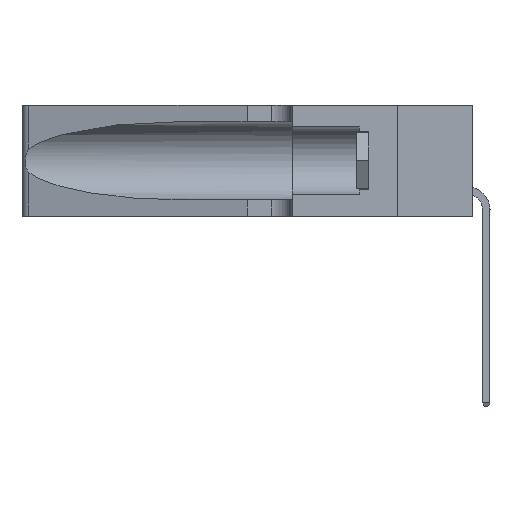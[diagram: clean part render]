
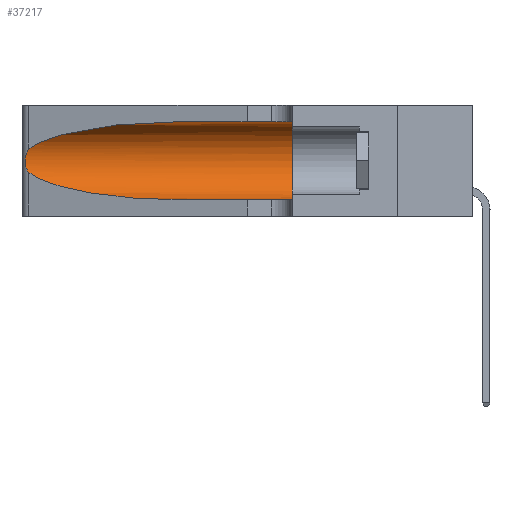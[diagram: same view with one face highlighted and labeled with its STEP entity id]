
A CAD part, left-side view. The second image highlights one B-rep face of the part: STEP entity #37217.
In plain terms, the highlighted cylindrical face has radius 3.308 mm (diameter 6.617 mm), a partial arc.
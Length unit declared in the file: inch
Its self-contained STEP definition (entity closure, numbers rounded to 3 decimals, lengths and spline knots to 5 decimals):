
#24 = CARTESIAN_POINT ( 'NONE',  ( 0.26075, 1.23896, 0.178 ) ) ;
#70 = CIRCLE ( 'NONE', #18635, 0.13025 ) ;
#520 = CARTESIAN_POINT ( 'NONE',  ( 0.1305, 1.61858, 0.31525 ) ) ;
#1106 = EDGE_CURVE ( 'NONE', #28408, #10484, #18541, .T. ) ;
#4346 = CARTESIAN_POINT ( 'NONE',  ( 0.18966, 0.96281, 0.31525 ) ) ;
#6622 = CARTESIAN_POINT ( 'NONE',  ( 0.1305, 0.35, 0.185 ) ) ;
#6805 = CARTESIAN_POINT ( 'NONE',  ( 0.25856, 1.23593, 0.16098 ) ) ;
#6912 = VERTEX_POINT ( 'NONE', #30365 ) ;
#6955 = CARTESIAN_POINT ( 'NONE',  ( 0.25487, 1.22718, 0.22369 ) ) ;
#7451 =( BOUNDED_CURVE ( )  B_SPLINE_CURVE ( 3, ( #17604, #4346, #10817, #21146 ),
 .UNSPECIFIED., .F., .F. ) 
 B_SPLINE_CURVE_WITH_KNOTS ( ( 4, 4 ),
 ( 1.5708, 2.84003 ),
 .UNSPECIFIED. ) 
 CURVE ( )  GEOMETRIC_REPRESENTATION_ITEM ( )  RATIONAL_B_SPLINE_CURVE ( ( 1., 0.87, 0.87, 1. ) ) 
 REPRESENTATION_ITEM ( '' )  );
#8233 = EDGE_CURVE ( 'NONE', #16642, #6912, #14654, .T. ) ;
#8557 =( BOUNDED_CURVE ( )  B_SPLINE_CURVE ( 3, ( #23113, #22842, #19428, #39682 ),
 .UNSPECIFIED., .F., .F. ) 
 B_SPLINE_CURVE_WITH_KNOTS ( ( 4, 4 ),
 ( 3.44316, 4.71239 ),
 .UNSPECIFIED. ) 
 CURVE ( )  GEOMETRIC_REPRESENTATION_ITEM ( )  RATIONAL_B_SPLINE_CURVE ( ( 1., 0.87, 0.87, 1. ) ) 
 REPRESENTATION_ITEM ( '' )  );
#9288 = CARTESIAN_POINT ( 'NONE',  ( 0.1305, 0.72297, 0.05475 ) ) ;
#10182 = CARTESIAN_POINT ( 'NONE',  ( 0.25555, 1.22993, 0.14849 ) ) ;
#10318 = CARTESIAN_POINT ( 'NONE',  ( 0.26018, 1.23835, 0.19895 ) ) ;
#10484 = VERTEX_POINT ( 'NONE', #36836 ) ;
#10817 = CARTESIAN_POINT ( 'NONE',  ( 0.2373, 1.15595, 0.28018 ) ) ;
#13384 = DIRECTION ( 'NONE',  ( 0., 0., 1. ) ) ;
#13590 = CARTESIAN_POINT ( 'NONE',  ( 0.25487, 1.22718, 0.14631 ) ) ;
#14347 = EDGE_CURVE ( 'NONE', #10484, #32507, #8557, .T. ) ;
#14654 = LINE ( 'NONE', #520, #37379 ) ;
#14724 = LINE ( 'NONE', #24856, #25330 ) ;
#16642 = VERTEX_POINT ( 'NONE', #31233 ) ;
#16738 = EDGE_CURVE ( 'NONE', #32507, #36580, #14724, .T. ) ;
#17604 = CARTESIAN_POINT ( 'NONE',  ( 0.1305, 0.72297, 0.31525 ) ) ;
#18541 = B_SPLINE_CURVE_WITH_KNOTS ( 'NONE', 3,
 ( #6955, #26858, #20503, #30702, #33678, #10318, #37094, #24, #23620, #6805, #43572, #30428, #10182, #13590 ),
 .UNSPECIFIED., .F., .F.,
 ( 4, 2, 2, 2, 2, 2, 4 ),
 ( 0., 0.00027, 0.00053, 0.00107, 0.0016, 0.00187, 0.00214 ),
 .UNSPECIFIED. ) ;
#18635 = AXIS2_PLACEMENT_3D ( 'NONE', #6622, #30216, #13384 ) ;
#19428 = CARTESIAN_POINT ( 'NONE',  ( 0.18966, 0.96281, 0.05475 ) ) ;
#19536 = CARTESIAN_POINT ( 'NONE',  ( 0.25487, 1.22718, 0.22369 ) ) ;
#20503 = CARTESIAN_POINT ( 'NONE',  ( 0.25639, 1.23184, 0.21858 ) ) ;
#20511 = ORIENTED_EDGE ( 'NONE', *, *, #8233, .F. ) ;
#21146 = CARTESIAN_POINT ( 'NONE',  ( 0.25487, 1.22718, 0.22369 ) ) ;
#21845 = EDGE_CURVE ( 'NONE', #6912, #36580, #70, .T. ) ;
#22668 = CARTESIAN_POINT ( 'NONE',  ( 0.1305, 1.61858, 0.185 ) ) ;
#22842 = CARTESIAN_POINT ( 'NONE',  ( 0.2373, 1.15595, 0.08982 ) ) ;
#23113 = CARTESIAN_POINT ( 'NONE',  ( 0.25487, 1.22718, 0.14631 ) ) ;
#23620 = CARTESIAN_POINT ( 'NONE',  ( 0.26017, 1.23833, 0.17102 ) ) ;
#24856 = CARTESIAN_POINT ( 'NONE',  ( 0.1305, 1.61858, 0.05475 ) ) ;
#25330 = VECTOR ( 'NONE', #34925, 39.37008 ) ;
#26858 = CARTESIAN_POINT ( 'NONE',  ( 0.25555, 1.22994, 0.2215 ) ) ;
#28408 = VERTEX_POINT ( 'NONE', #19536 ) ;
#29611 = ORIENTED_EDGE ( 'NONE', *, *, #14347, .T. ) ;
#30092 = ORIENTED_EDGE ( 'NONE', *, *, #21845, .F. ) ;
#30216 = DIRECTION ( 'NONE',  ( 0., 1., 0. ) ) ;
#30365 = CARTESIAN_POINT ( 'NONE',  ( 0.1305, 0.35, 0.31525 ) ) ;
#30428 = CARTESIAN_POINT ( 'NONE',  ( 0.25639, 1.23186, 0.15144 ) ) ;
#30702 = CARTESIAN_POINT ( 'NONE',  ( 0.25787, 1.23484, 0.2124 ) ) ;
#31233 = CARTESIAN_POINT ( 'NONE',  ( 0.1305, 0.72297, 0.31525 ) ) ;
#31606 = ORIENTED_EDGE ( 'NONE', *, *, #16738, .T. ) ;
#32291 = EDGE_LOOP ( 'NONE', ( #36996, #38528, #29611, #31606, #30092, #20511 ) ) ;
#32507 = VERTEX_POINT ( 'NONE', #9288 ) ;
#33678 = CARTESIAN_POINT ( 'NONE',  ( 0.25854, 1.2359, 0.20912 ) ) ;
#34925 = DIRECTION ( 'NONE',  ( 0., -1., 0. ) ) ;
#35882 = CARTESIAN_POINT ( 'NONE',  ( 0.1305, 0.35, 0.05475 ) ) ;
#36580 = VERTEX_POINT ( 'NONE', #35882 ) ;
#36836 = CARTESIAN_POINT ( 'NONE',  ( 0.25487, 1.22718, 0.14631 ) ) ;
#36996 = ORIENTED_EDGE ( 'NONE', *, *, #43407, .T. ) ;
#37094 = CARTESIAN_POINT ( 'NONE',  ( 0.26075, 1.23896, 0.19203 ) ) ;
#37217 = ADVANCED_FACE ( 'NONE', ( #40666 ), #37495, .F. ) ;
#37379 = VECTOR ( 'NONE', #40546, 39.37008 ) ;
#37495 = CYLINDRICAL_SURFACE ( 'NONE', #42348, 0.13025 ) ;
#38528 = ORIENTED_EDGE ( 'NONE', *, *, #1106, .T. ) ;
#39649 = DIRECTION ( 'NONE',  ( 0., 0., -1. ) ) ;
#39682 = CARTESIAN_POINT ( 'NONE',  ( 0.1305, 0.72297, 0.05475 ) ) ;
#40546 = DIRECTION ( 'NONE',  ( 0., -1., 0. ) ) ;
#40666 = FACE_OUTER_BOUND ( 'NONE', #32291, .T. ) ;
#42348 = AXIS2_PLACEMENT_3D ( 'NONE', #22668, #43068, #39649 ) ;
#43068 = DIRECTION ( 'NONE',  ( 0., -1., 0. ) ) ;
#43407 = EDGE_CURVE ( 'NONE', #16642, #28408, #7451, .T. ) ;
#43572 = CARTESIAN_POINT ( 'NONE',  ( 0.25789, 1.23486, 0.15765 ) ) ;
